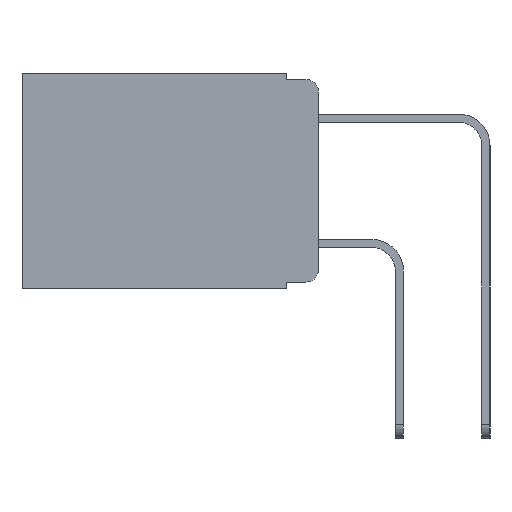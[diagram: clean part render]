
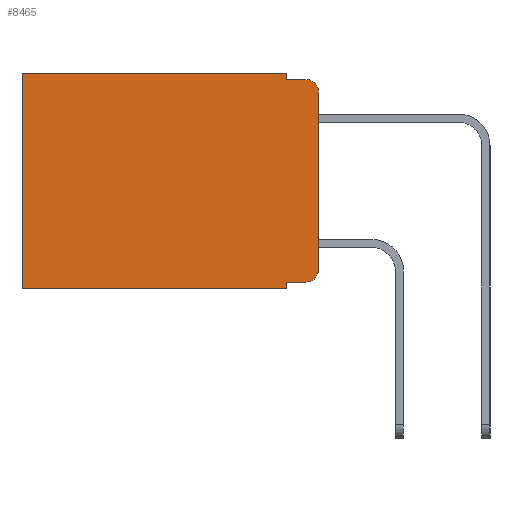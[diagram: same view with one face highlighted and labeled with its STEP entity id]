
A CAD part, left-side view. The second image highlights one B-rep face of the part: STEP entity #8465.
In plain terms, the highlighted planar face has unit normal (-1, 0, 0).
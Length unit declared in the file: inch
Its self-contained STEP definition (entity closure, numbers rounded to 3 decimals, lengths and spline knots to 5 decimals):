
#51 = VERTEX_POINT ( 'NONE', #11004 ) ;
#265 = VECTOR ( 'NONE', #19419, 39.37008 ) ;
#475 = CIRCLE ( 'NONE', #17119, 0.02 ) ;
#809 = DIRECTION ( 'NONE',  ( -1., 0., 0. ) ) ;
#893 = ORIENTED_EDGE ( 'NONE', *, *, #14559, .T. ) ;
#931 = LINE ( 'NONE', #7103, #265 ) ;
#1245 = ORIENTED_EDGE ( 'NONE', *, *, #6053, .T. ) ;
#1427 = VERTEX_POINT ( 'NONE', #20294 ) ;
#1680 = EDGE_CURVE ( 'NONE', #3238, #4234, #17475, .T. ) ;
#2225 = ORIENTED_EDGE ( 'NONE', *, *, #12688, .F. ) ;
#2768 = DIRECTION ( 'NONE',  ( 0., 0., -1. ) ) ;
#3095 = CARTESIAN_POINT ( 'NONE',  ( 0.298, 0.473, 0. ) ) ;
#3236 = LINE ( 'NONE', #6516, #14422 ) ;
#3238 = VERTEX_POINT ( 'NONE', #5861 ) ;
#3782 = VERTEX_POINT ( 'NONE', #10112 ) ;
#4234 = VERTEX_POINT ( 'NONE', #6734 ) ;
#4254 = ORIENTED_EDGE ( 'NONE', *, *, #17304, .F. ) ;
#4352 = VECTOR ( 'NONE', #24147, 39.37008 ) ;
#5229 = EDGE_CURVE ( 'NONE', #22179, #23365, #17613, .T. ) ;
#5357 = VECTOR ( 'NONE', #18448, 39.37008 ) ;
#5478 = EDGE_LOOP ( 'NONE', ( #16906, #893, #12162, #2225, #9228, #20032, #4254, #21266, #5620, #1245 ) ) ;
#5620 = ORIENTED_EDGE ( 'NONE', *, *, #24626, .T. ) ;
#5861 = CARTESIAN_POINT ( 'NONE',  ( 0.298, 0., -0.03 ) ) ;
#6053 = EDGE_CURVE ( 'NONE', #25184, #4234, #10558, .T. ) ;
#6516 = CARTESIAN_POINT ( 'NONE',  ( 0.298, 0.473, 0. ) ) ;
#6529 = VECTOR ( 'NONE', #2768, 39.37008 ) ;
#6734 = CARTESIAN_POINT ( 'NONE',  ( 0.298, 0., -0.313 ) ) ;
#7103 = CARTESIAN_POINT ( 'NONE',  ( 0.298, 0.051, 0. ) ) ;
#7216 = CARTESIAN_POINT ( 'NONE',  ( 0.298, 0.051, 0. ) ) ;
#7468 = VECTOR ( 'NONE', #23455, 39.37008 ) ;
#7842 = CARTESIAN_POINT ( 'NONE',  ( 0.298, 0., 0. ) ) ;
#7937 = CARTESIAN_POINT ( 'NONE',  ( 0.298, 0.051, -0.333 ) ) ;
#8465 = ADVANCED_FACE ( 'NONE', ( #15753 ), #8594, .F. ) ;
#8561 = CARTESIAN_POINT ( 'NONE',  ( 0.298, 0., 0. ) ) ;
#8594 = PLANE ( 'NONE',  #10532 ) ;
#9055 = DIRECTION ( 'NONE',  ( -1., 0., 0. ) ) ;
#9228 = ORIENTED_EDGE ( 'NONE', *, *, #5229, .T. ) ;
#9958 = EDGE_CURVE ( 'NONE', #23365, #20838, #3236, .T. ) ;
#10091 = CARTESIAN_POINT ( 'NONE',  ( 0.298, 0.02, -0.333 ) ) ;
#10112 = CARTESIAN_POINT ( 'NONE',  ( 0.298, 0.02, -0.01 ) ) ;
#10532 = AXIS2_PLACEMENT_3D ( 'NONE', #8561, #19315, #18513 ) ;
#10558 = CIRCLE ( 'NONE', #14620, 0.02 ) ;
#11004 = CARTESIAN_POINT ( 'NONE',  ( 0.298, 0.051, -0.01 ) ) ;
#11173 = CARTESIAN_POINT ( 'NONE',  ( 0.298, 0.02, -0.313 ) ) ;
#11599 = LINE ( 'NONE', #22340, #5357 ) ;
#12162 = ORIENTED_EDGE ( 'NONE', *, *, #17262, .F. ) ;
#12688 = EDGE_CURVE ( 'NONE', #22179, #51, #23644, .T. ) ;
#12855 = VECTOR ( 'NONE', #22039, 39.37008 ) ;
#13468 = CARTESIAN_POINT ( 'NONE',  ( 0.298, 0.02, -0.03 ) ) ;
#14422 = VECTOR ( 'NONE', #20775, 39.37008 ) ;
#14559 = EDGE_CURVE ( 'NONE', #3238, #3782, #475, .T. ) ;
#14620 = AXIS2_PLACEMENT_3D ( 'NONE', #11173, #9055, #23207 ) ;
#15102 = VECTOR ( 'NONE', #16511, 39.37008 ) ;
#15488 = DIRECTION ( 'NONE',  ( 0., 0., -1. ) ) ;
#15508 = CARTESIAN_POINT ( 'NONE',  ( 0.298, 0.051, 0. ) ) ;
#15753 = FACE_OUTER_BOUND ( 'NONE', #5478, .T. ) ;
#16511 = DIRECTION ( 'NONE',  ( 0., 1., 0. ) ) ;
#16906 = ORIENTED_EDGE ( 'NONE', *, *, #1680, .F. ) ;
#17119 = AXIS2_PLACEMENT_3D ( 'NONE', #13468, #809, #15488 ) ;
#17262 = EDGE_CURVE ( 'NONE', #51, #3782, #11599, .T. ) ;
#17304 = EDGE_CURVE ( 'NONE', #1427, #20838, #25730, .T. ) ;
#17475 = LINE ( 'NONE', #17794, #6529 ) ;
#17613 = LINE ( 'NONE', #7842, #12855 ) ;
#17794 = CARTESIAN_POINT ( 'NONE',  ( 0.298, 0., 0. ) ) ;
#18096 = EDGE_CURVE ( 'NONE', #22948, #1427, #931, .T. ) ;
#18448 = DIRECTION ( 'NONE',  ( 0., -1., 0. ) ) ;
#18513 = DIRECTION ( 'NONE',  ( 0., 0., -1. ) ) ;
#19315 = DIRECTION ( 'NONE',  ( 1., 0., 0. ) ) ;
#19419 = DIRECTION ( 'NONE',  ( 0., 0., -1. ) ) ;
#20032 = ORIENTED_EDGE ( 'NONE', *, *, #9958, .T. ) ;
#20294 = CARTESIAN_POINT ( 'NONE',  ( 0.298, 0.051, -0.343 ) ) ;
#20775 = DIRECTION ( 'NONE',  ( 0., 0., -1. ) ) ;
#20838 = VERTEX_POINT ( 'NONE', #21637 ) ;
#21266 = ORIENTED_EDGE ( 'NONE', *, *, #18096, .F. ) ;
#21637 = CARTESIAN_POINT ( 'NONE',  ( 0.298, 0.473, -0.343 ) ) ;
#22039 = DIRECTION ( 'NONE',  ( 0., 1., 0. ) ) ;
#22179 = VERTEX_POINT ( 'NONE', #15508 ) ;
#22340 = CARTESIAN_POINT ( 'NONE',  ( 0.298, 0.051, -0.01 ) ) ;
#22508 = CARTESIAN_POINT ( 'NONE',  ( 0.298, 0., -0.343 ) ) ;
#22948 = VERTEX_POINT ( 'NONE', #23955 ) ;
#23207 = DIRECTION ( 'NONE',  ( 0., 0., -1. ) ) ;
#23365 = VERTEX_POINT ( 'NONE', #3095 ) ;
#23455 = DIRECTION ( 'NONE',  ( 0., 0., -1. ) ) ;
#23644 = LINE ( 'NONE', #7216, #7468 ) ;
#23955 = CARTESIAN_POINT ( 'NONE',  ( 0.298, 0.051, -0.333 ) ) ;
#24147 = DIRECTION ( 'NONE',  ( 0., -1., 0. ) ) ;
#24626 = EDGE_CURVE ( 'NONE', #22948, #25184, #25440, .T. ) ;
#25184 = VERTEX_POINT ( 'NONE', #10091 ) ;
#25440 = LINE ( 'NONE', #7937, #4352 ) ;
#25730 = LINE ( 'NONE', #22508, #15102 ) ;
